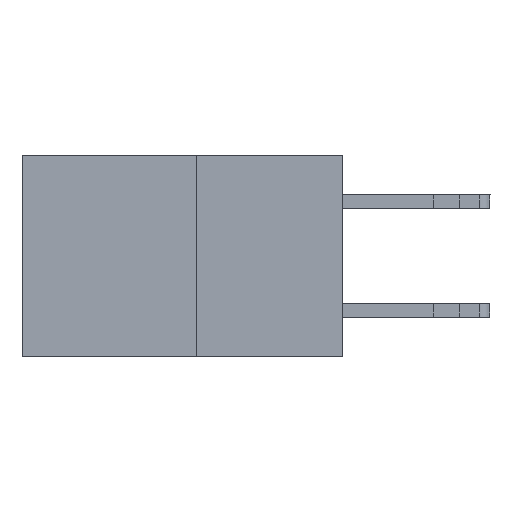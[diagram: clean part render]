
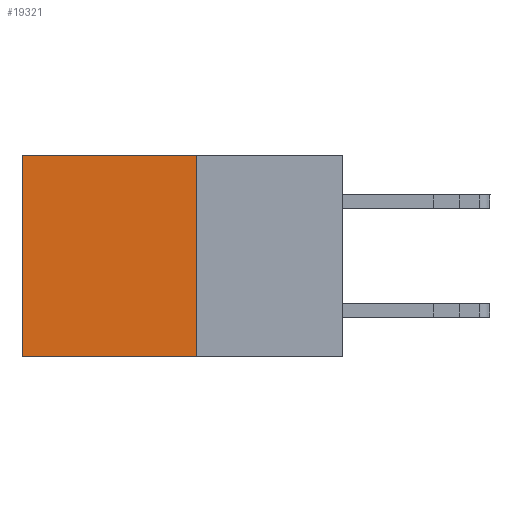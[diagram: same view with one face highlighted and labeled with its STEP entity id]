
A CAD part, left-side view. The second image highlights one B-rep face of the part: STEP entity #19321.
In plain terms, the highlighted planar face has unit normal (-1, 0, 0).
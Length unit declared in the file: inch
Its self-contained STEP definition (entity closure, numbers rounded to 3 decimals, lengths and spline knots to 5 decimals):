
#678 = VECTOR ( 'NONE', #4660, 39.37008 ) ;
#891 = LINE ( 'NONE', #14014, #18717 ) ;
#2147 = EDGE_CURVE ( 'NONE', #8154, #20744, #7269, .T. ) ;
#2301 = DIRECTION ( 'NONE',  ( 1., 0., 0. ) ) ;
#4318 = EDGE_CURVE ( 'NONE', #15499, #15160, #6068, .T. ) ;
#4660 = DIRECTION ( 'NONE',  ( 0., 1., 0. ) ) ;
#5072 = LINE ( 'NONE', #18363, #14117 ) ;
#5423 = CARTESIAN_POINT ( 'NONE',  ( 0.277, 0.27, -0.37 ) ) ;
#5885 = CARTESIAN_POINT ( 'NONE',  ( 0.277, 0.59, -0.37 ) ) ;
#6068 = LINE ( 'NONE', #9193, #678 ) ;
#7269 = LINE ( 'NONE', #20447, #18818 ) ;
#8154 = VERTEX_POINT ( 'NONE', #11413 ) ;
#8564 = DIRECTION ( 'NONE',  ( 0., 0., -1. ) ) ;
#8713 = DIRECTION ( 'NONE',  ( 0., 0., -1. ) ) ;
#9193 = CARTESIAN_POINT ( 'NONE',  ( 0.277, 0.27, -0.37 ) ) ;
#9196 = DIRECTION ( 'NONE',  ( 0., 0., -1. ) ) ;
#10384 = ORIENTED_EDGE ( 'NONE', *, *, #17881, .T. ) ;
#10578 = CARTESIAN_POINT ( 'NONE',  ( 0.277, 0.59, 0. ) ) ;
#11413 = CARTESIAN_POINT ( 'NONE',  ( 0.277, 0.27, 0. ) ) ;
#11966 = PLANE ( 'NONE',  #12628 ) ;
#12051 = ORIENTED_EDGE ( 'NONE', *, *, #20243, .F. ) ;
#12628 = AXIS2_PLACEMENT_3D ( 'NONE', #13498, #2301, #8564 ) ;
#13498 = CARTESIAN_POINT ( 'NONE',  ( 0.277, 0.27, -0.37 ) ) ;
#14014 = CARTESIAN_POINT ( 'NONE',  ( 0.277, 0.59, -0.37 ) ) ;
#14117 = VECTOR ( 'NONE', #8713, 39.37008 ) ;
#15160 = VERTEX_POINT ( 'NONE', #5885 ) ;
#15499 = VERTEX_POINT ( 'NONE', #5423 ) ;
#17029 = DIRECTION ( 'NONE',  ( 0., 1., 0. ) ) ;
#17881 = EDGE_CURVE ( 'NONE', #20744, #15160, #891, .T. ) ;
#18363 = CARTESIAN_POINT ( 'NONE',  ( 0.277, 0.27, -0.37 ) ) ;
#18503 = FACE_OUTER_BOUND ( 'NONE', #20295, .T. ) ;
#18717 = VECTOR ( 'NONE', #9196, 39.37008 ) ;
#18818 = VECTOR ( 'NONE', #17029, 39.37008 ) ;
#19321 = ADVANCED_FACE ( 'NONE', ( #18503 ), #11966, .F. ) ;
#20224 = ORIENTED_EDGE ( 'NONE', *, *, #2147, .T. ) ;
#20243 = EDGE_CURVE ( 'NONE', #8154, #15499, #5072, .T. ) ;
#20295 = EDGE_LOOP ( 'NONE', ( #10384, #20339, #12051, #20224 ) ) ;
#20339 = ORIENTED_EDGE ( 'NONE', *, *, #4318, .F. ) ;
#20447 = CARTESIAN_POINT ( 'NONE',  ( 0.277, 0.27, 0. ) ) ;
#20744 = VERTEX_POINT ( 'NONE', #10578 ) ;
